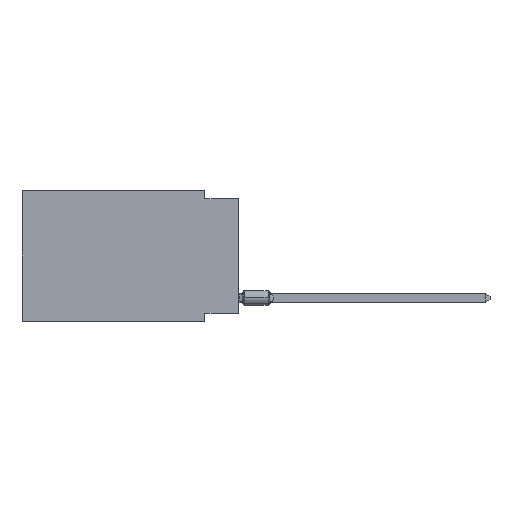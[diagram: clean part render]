
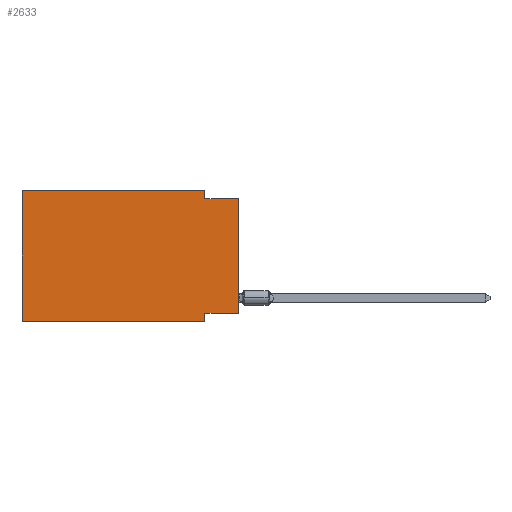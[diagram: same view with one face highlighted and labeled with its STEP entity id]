
A CAD part, left-side view. The second image highlights one B-rep face of the part: STEP entity #2633.
In plain terms, the highlighted planar face has unit normal (-1, 0, 0).
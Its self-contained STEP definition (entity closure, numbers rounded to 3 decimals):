
#994 = DIRECTION ( 'NONE',  ( 0., 0., 1. ) ) ;
#1265 = DIRECTION ( 'NONE',  ( 1., 0., 0. ) ) ;
#1325 = EDGE_CURVE ( 'NONE', #1707, #16095, #4491, .T. ) ;
#1707 = VERTEX_POINT ( 'NONE', #19026 ) ;
#2038 = ORIENTED_EDGE ( 'NONE', *, *, #15596, .F. ) ;
#2474 = VERTEX_POINT ( 'NONE', #6582 ) ;
#2633 = ADVANCED_FACE ( 'NONE', ( #9643 ), #16024, .F. ) ;
#3336 = LINE ( 'NONE', #19468, #11713 ) ;
#4050 = VECTOR ( 'NONE', #16674, 1000. ) ;
#4453 = CARTESIAN_POINT ( 'NONE',  ( 0., 2.54, 0. ) ) ;
#4491 = LINE ( 'NONE', #10992, #17167 ) ;
#4564 = ORIENTED_EDGE ( 'NONE', *, *, #18555, .F. ) ;
#5162 = VERTEX_POINT ( 'NONE', #8249 ) ;
#5388 = ORIENTED_EDGE ( 'NONE', *, *, #13996, .T. ) ;
#5884 = EDGE_CURVE ( 'NONE', #12023, #1707, #19902, .T. ) ;
#6433 = ORIENTED_EDGE ( 'NONE', *, *, #13559, .F. ) ;
#6582 = CARTESIAN_POINT ( 'NONE',  ( 0., 16.383, 0. ) ) ;
#6897 = CARTESIAN_POINT ( 'NONE',  ( 0., 2.54, -0.635 ) ) ;
#7056 = DIRECTION ( 'NONE',  ( 0., 1., 0. ) ) ;
#7879 = DIRECTION ( 'NONE',  ( 0., -1., 0. ) ) ;
#7933 = CARTESIAN_POINT ( 'NONE',  ( 0., 2.54, -9.906 ) ) ;
#8249 = CARTESIAN_POINT ( 'NONE',  ( 0., 16.383, -9.906 ) ) ;
#8912 = CARTESIAN_POINT ( 'NONE',  ( 0., 16.383, 0. ) ) ;
#9065 = CARTESIAN_POINT ( 'NONE',  ( 0., 0., 0. ) ) ;
#9481 = VECTOR ( 'NONE', #14935, 1000. ) ;
#9507 = DIRECTION ( 'NONE',  ( 0., 0., 1. ) ) ;
#9643 = FACE_OUTER_BOUND ( 'NONE', #10799, .T. ) ;
#9793 = VECTOR ( 'NONE', #994, 1000. ) ;
#10246 = VERTEX_POINT ( 'NONE', #16762 ) ;
#10799 = EDGE_LOOP ( 'NONE', ( #18223, #15106, #2038, #4564, #6433, #5388, #13522, #13547 ) ) ;
#10872 = LINE ( 'NONE', #12565, #14205 ) ;
#10992 = CARTESIAN_POINT ( 'NONE',  ( 0., 2.54, -9.906 ) ) ;
#11028 = CARTESIAN_POINT ( 'NONE',  ( 0., 16.383, 0. ) ) ;
#11259 = VERTEX_POINT ( 'NONE', #4453 ) ;
#11391 = VECTOR ( 'NONE', #7879, 1000. ) ;
#11641 = LINE ( 'NONE', #18101, #9481 ) ;
#11713 = VECTOR ( 'NONE', #9507, 1000. ) ;
#11734 = CARTESIAN_POINT ( 'NONE',  ( 0., 0., -9.271 ) ) ;
#12023 = VERTEX_POINT ( 'NONE', #16223 ) ;
#12565 = CARTESIAN_POINT ( 'NONE',  ( 0., 2.54, 0. ) ) ;
#13522 = ORIENTED_EDGE ( 'NONE', *, *, #1325, .F. ) ;
#13547 = ORIENTED_EDGE ( 'NONE', *, *, #5884, .F. ) ;
#13559 = EDGE_CURVE ( 'NONE', #5162, #2474, #3336, .T. ) ;
#13996 = EDGE_CURVE ( 'NONE', #5162, #16095, #15960, .T. ) ;
#14205 = VECTOR ( 'NONE', #18617, 1000. ) ;
#14935 = DIRECTION ( 'NONE',  ( 0., -1., 0. ) ) ;
#15106 = ORIENTED_EDGE ( 'NONE', *, *, #18904, .F. ) ;
#15126 = EDGE_CURVE ( 'NONE', #12023, #10246, #17032, .T. ) ;
#15285 = VECTOR ( 'NONE', #7056, 1000. ) ;
#15596 = EDGE_CURVE ( 'NONE', #11259, #19662, #10872, .T. ) ;
#15960 = LINE ( 'NONE', #19442, #11391 ) ;
#16024 = PLANE ( 'NONE',  #19244 ) ;
#16095 = VERTEX_POINT ( 'NONE', #7933 ) ;
#16124 = DIRECTION ( 'NONE',  ( 0., 0., -1. ) ) ;
#16223 = CARTESIAN_POINT ( 'NONE',  ( 0., 0., -9.271 ) ) ;
#16674 = DIRECTION ( 'NONE',  ( 0., -1., 0. ) ) ;
#16762 = CARTESIAN_POINT ( 'NONE',  ( 0., 0., -0.635 ) ) ;
#16990 = LINE ( 'NONE', #8912, #4050 ) ;
#17032 = LINE ( 'NONE', #9065, #9793 ) ;
#17167 = VECTOR ( 'NONE', #17453, 1000. ) ;
#17453 = DIRECTION ( 'NONE',  ( 0., 0., -1. ) ) ;
#18101 = CARTESIAN_POINT ( 'NONE',  ( 0., 0., -0.635 ) ) ;
#18223 = ORIENTED_EDGE ( 'NONE', *, *, #15126, .T. ) ;
#18555 = EDGE_CURVE ( 'NONE', #2474, #11259, #16990, .T. ) ;
#18617 = DIRECTION ( 'NONE',  ( 0., 0., -1. ) ) ;
#18904 = EDGE_CURVE ( 'NONE', #19662, #10246, #11641, .T. ) ;
#19026 = CARTESIAN_POINT ( 'NONE',  ( 0., 2.54, -9.271 ) ) ;
#19244 = AXIS2_PLACEMENT_3D ( 'NONE', #11028, #1265, #16124 ) ;
#19442 = CARTESIAN_POINT ( 'NONE',  ( 0., 16.383, -9.906 ) ) ;
#19468 = CARTESIAN_POINT ( 'NONE',  ( 0., 16.383, 0. ) ) ;
#19662 = VERTEX_POINT ( 'NONE', #6897 ) ;
#19902 = LINE ( 'NONE', #11734, #15285 ) ;
